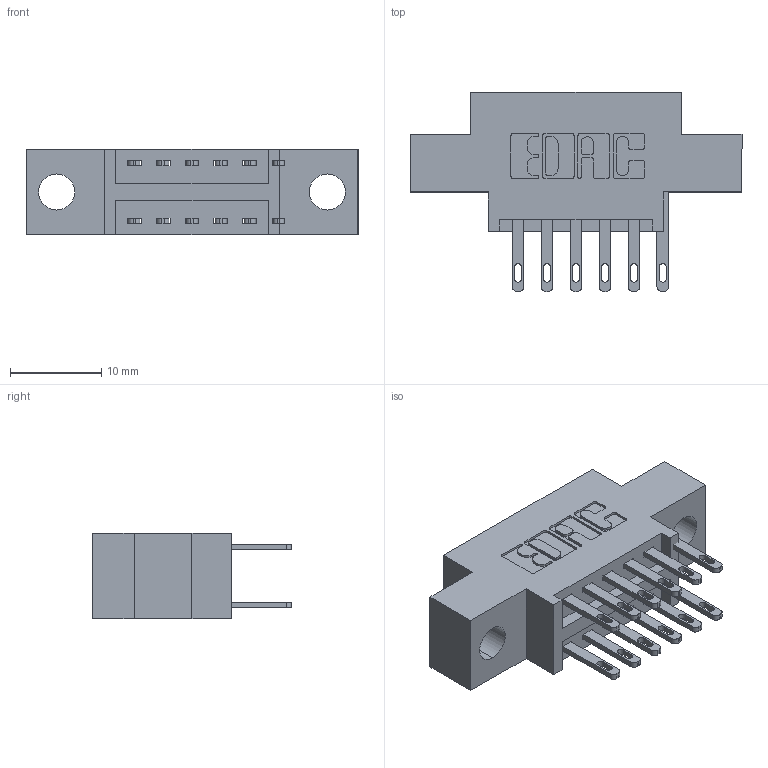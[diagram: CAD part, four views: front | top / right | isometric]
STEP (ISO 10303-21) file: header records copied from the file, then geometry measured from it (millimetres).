
FILE_DESCRIPTION (( 'STEP AP203' ), '1' );
FILE_NAME ('346-012-500-804.STEP', '2022-05-17T18:54:38', ( '' ), ( '' ), 'SwSTEP 2.0', 'SolidWorks 2020', '' );
FILE_SCHEMA (( 'CONFIG_CONTROL_DESIGN' ));
Length unit declared in the file: inch
Products named in the file (3): 345-292-001_345-293-100; 346-012-500-804; 346 Part_0.170 Offset - 0.156 Dia-TH
Assembly tree (13 placements, depth 2):
  346-012-500-804
    346 Part_0.170 Offset - 0.156 Dia-TH
    345-292-001_345-293-100  x12
Bounding box: 36.45 x 21.84 x 9.4 mm (x, y, z)
Volume: 3061 mm3; surface area: 3882.9 mm2
Topology: 13 solids, 13 shells, 704 faces, 2099 edges, 1398 vertices
Faces by surface type: plane 432, cylinder 272
Entity records: 8789 total; most frequent: CARTESIAN_POINT 1496, ORIENTED_EDGE 1426, DIRECTION 1373, EDGE_CURVE 713, LINE 557, VECTOR 557, VERTEX_POINT 474, AXIS2_PLACEMENT_3D 408
